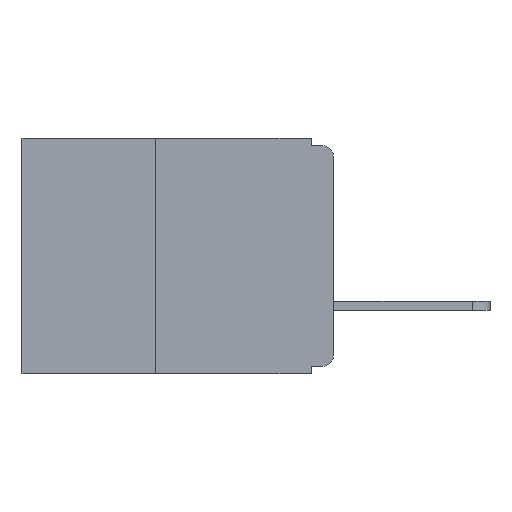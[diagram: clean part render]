
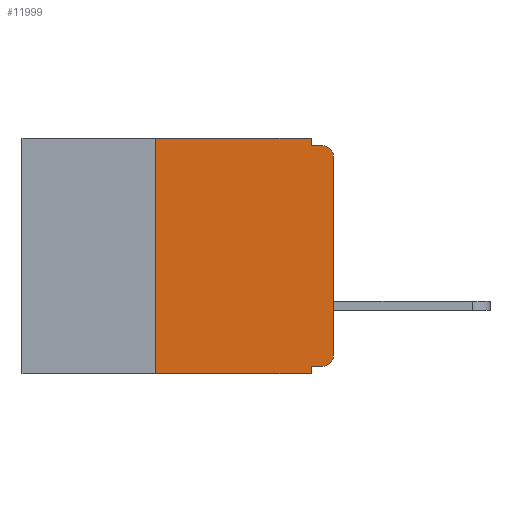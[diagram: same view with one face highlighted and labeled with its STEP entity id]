
A CAD part, left-side view. The second image highlights one B-rep face of the part: STEP entity #11999.
In plain terms, the highlighted planar face has unit normal (-1, 0, 0).
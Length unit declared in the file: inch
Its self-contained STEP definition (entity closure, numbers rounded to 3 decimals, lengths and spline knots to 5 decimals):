
#208 = EDGE_CURVE ( 'NONE', #11726, #12255, #2124, .T. ) ;
#906 = FACE_OUTER_BOUND ( 'NONE', #6678, .T. ) ;
#1423 = ORIENTED_EDGE ( 'NONE', *, *, #208, .T. ) ;
#1496 = VERTEX_POINT ( 'NONE', #15829 ) ;
#1510 = ORIENTED_EDGE ( 'NONE', *, *, #8678, .F. ) ;
#1636 = EDGE_CURVE ( 'NONE', #11771, #15073, #14547, .T. ) ;
#1670 = CARTESIAN_POINT ( 'NONE',  ( 0., 0., -0.025 ) ) ;
#2124 = CIRCLE ( 'NONE', #14065, 0.015 ) ;
#2882 = ORIENTED_EDGE ( 'NONE', *, *, #15389, .F. ) ;
#3361 = ORIENTED_EDGE ( 'NONE', *, *, #14051, .T. ) ;
#3444 = EDGE_CURVE ( 'NONE', #17876, #15811, #9443, .T. ) ;
#3721 = VERTEX_POINT ( 'NONE', #6592 ) ;
#4026 = VERTEX_POINT ( 'NONE', #13930 ) ;
#4395 = ORIENTED_EDGE ( 'NONE', *, *, #17927, .F. ) ;
#4425 = DIRECTION ( 'NONE',  ( 0., -1., 0. ) ) ;
#4910 = DIRECTION ( 'NONE',  ( 0., 1., 0. ) ) ;
#5056 = CARTESIAN_POINT ( 'NONE',  ( 0., 0., -0.32 ) ) ;
#5383 = VECTOR ( 'NONE', #9858, 39.37008 ) ;
#5463 = CARTESIAN_POINT ( 'NONE',  ( 0., 0.437, 0. ) ) ;
#5909 = LINE ( 'NONE', #9068, #5383 ) ;
#6347 = CARTESIAN_POINT ( 'NONE',  ( 0., 0.25, 0. ) ) ;
#6351 = VERTEX_POINT ( 'NONE', #8040 ) ;
#6592 = CARTESIAN_POINT ( 'NONE',  ( 0., 0.25, -0.33 ) ) ;
#6678 = EDGE_LOOP ( 'NONE', ( #3361, #1423, #2882, #14631, #15055, #15639, #16645, #1510, #4395, #7937 ) ) ;
#7937 = ORIENTED_EDGE ( 'NONE', *, *, #1636, .T. ) ;
#7946 = DIRECTION ( 'NONE',  ( 0., 0., -1. ) ) ;
#8013 = CARTESIAN_POINT ( 'NONE',  ( 0., 0.031, -0.33 ) ) ;
#8040 = CARTESIAN_POINT ( 'NONE',  ( 0., 0.031, -0.33 ) ) ;
#8129 = EDGE_CURVE ( 'NONE', #15811, #1496, #13810, .T. ) ;
#8351 = CARTESIAN_POINT ( 'NONE',  ( 0., 0.031, 0. ) ) ;
#8503 = EDGE_CURVE ( 'NONE', #3721, #17876, #12954, .T. ) ;
#8538 = EDGE_CURVE ( 'NONE', #3721, #6351, #12894, .T. ) ;
#8678 = EDGE_CURVE ( 'NONE', #4026, #6351, #12458, .T. ) ;
#9068 = CARTESIAN_POINT ( 'NONE',  ( 0., 0., 0. ) ) ;
#9302 = VECTOR ( 'NONE', #4425, 39.37008 ) ;
#9443 = LINE ( 'NONE', #5463, #9302 ) ;
#9818 = CARTESIAN_POINT ( 'NONE',  ( 0., 0.015, -0.025 ) ) ;
#9858 = DIRECTION ( 'NONE',  ( 0., 0., 1. ) ) ;
#9922 = DIRECTION ( 'NONE',  ( 0., -1., 0. ) ) ;
#10030 = DIRECTION ( 'NONE',  ( 0., 0., -1. ) ) ;
#10098 = DIRECTION ( 'NONE',  ( 1., 0., 0. ) ) ;
#10142 = CARTESIAN_POINT ( 'NONE',  ( 0., 0.437, -0.33 ) ) ;
#10283 = DIRECTION ( 'NONE',  ( 0., 0., 1. ) ) ;
#10285 = DIRECTION ( 'NONE',  ( 0., 0., -1. ) ) ;
#10395 = CARTESIAN_POINT ( 'NONE',  ( 0., 0.437, 0. ) ) ;
#10433 = DIRECTION ( 'NONE',  ( -1., 0., 0. ) ) ;
#10450 = CARTESIAN_POINT ( 'NONE',  ( 0., 0.015, -0.305 ) ) ;
#10694 = CARTESIAN_POINT ( 'NONE',  ( 0., 0.25, -0.33 ) ) ;
#10744 = AXIS2_PLACEMENT_3D ( 'NONE', #10450, #10433, #10285 ) ;
#11275 = DIRECTION ( 'NONE',  ( 0., -1., 0. ) ) ;
#11379 = PLANE ( 'NONE',  #11969 ) ;
#11382 = CARTESIAN_POINT ( 'NONE',  ( 0., 0., -0.01 ) ) ;
#11726 = VERTEX_POINT ( 'NONE', #1670 ) ;
#11771 = VERTEX_POINT ( 'NONE', #14077 ) ;
#11969 = AXIS2_PLACEMENT_3D ( 'NONE', #10395, #10098, #10030 ) ;
#11999 = ADVANCED_FACE ( 'NONE', ( #906 ), #11379, .F. ) ;
#12255 = VERTEX_POINT ( 'NONE', #16482 ) ;
#12458 = LINE ( 'NONE', #8013, #12607 ) ;
#12607 = VECTOR ( 'NONE', #7946, 39.37008 ) ;
#12878 = VECTOR ( 'NONE', #9922, 39.37008 ) ;
#12894 = LINE ( 'NONE', #10142, #12878 ) ;
#12935 = VECTOR ( 'NONE', #10283, 39.37008 ) ;
#12954 = LINE ( 'NONE', #10694, #12935 ) ;
#13753 = VECTOR ( 'NONE', #15240, 39.37008 ) ;
#13810 = LINE ( 'NONE', #15431, #13753 ) ;
#13930 = CARTESIAN_POINT ( 'NONE',  ( 0., 0.031, -0.32 ) ) ;
#14047 = DIRECTION ( 'NONE',  ( 0., 0., -1. ) ) ;
#14051 = EDGE_CURVE ( 'NONE', #15073, #11726, #5909, .T. ) ;
#14065 = AXIS2_PLACEMENT_3D ( 'NONE', #9818, #14302, #14047 ) ;
#14077 = CARTESIAN_POINT ( 'NONE',  ( 0., 0.015, -0.32 ) ) ;
#14302 = DIRECTION ( 'NONE',  ( -1., 0., 0. ) ) ;
#14547 = CIRCLE ( 'NONE', #10744, 0.015 ) ;
#14631 = ORIENTED_EDGE ( 'NONE', *, *, #8129, .F. ) ;
#15055 = ORIENTED_EDGE ( 'NONE', *, *, #3444, .F. ) ;
#15073 = VERTEX_POINT ( 'NONE', #16665 ) ;
#15240 = DIRECTION ( 'NONE',  ( 0., 0., -1. ) ) ;
#15389 = EDGE_CURVE ( 'NONE', #1496, #12255, #17900, .T. ) ;
#15431 = CARTESIAN_POINT ( 'NONE',  ( 0., 0.031, 0. ) ) ;
#15461 = VECTOR ( 'NONE', #4910, 39.37008 ) ;
#15639 = ORIENTED_EDGE ( 'NONE', *, *, #8503, .F. ) ;
#15811 = VERTEX_POINT ( 'NONE', #8351 ) ;
#15829 = CARTESIAN_POINT ( 'NONE',  ( 0., 0.031, -0.01 ) ) ;
#16136 = LINE ( 'NONE', #5056, #15461 ) ;
#16482 = CARTESIAN_POINT ( 'NONE',  ( 0., 0.015, -0.01 ) ) ;
#16645 = ORIENTED_EDGE ( 'NONE', *, *, #8538, .T. ) ;
#16665 = CARTESIAN_POINT ( 'NONE',  ( 0., 0., -0.305 ) ) ;
#17776 = VECTOR ( 'NONE', #11275, 39.37008 ) ;
#17876 = VERTEX_POINT ( 'NONE', #6347 ) ;
#17900 = LINE ( 'NONE', #11382, #17776 ) ;
#17927 = EDGE_CURVE ( 'NONE', #11771, #4026, #16136, .T. ) ;
